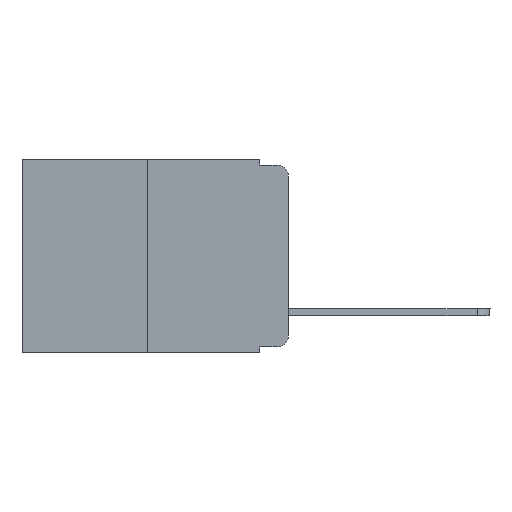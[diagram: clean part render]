
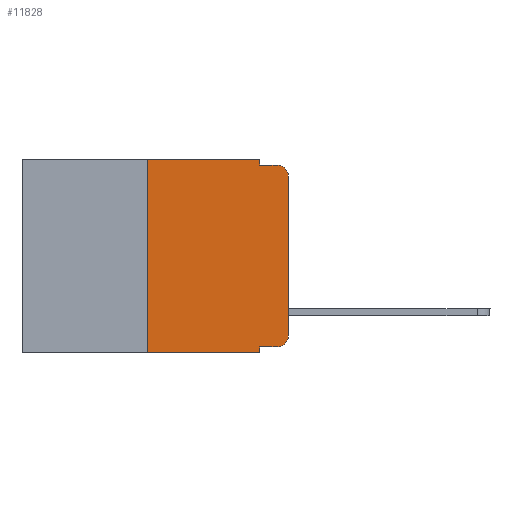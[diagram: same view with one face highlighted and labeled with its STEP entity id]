
A CAD part, left-side view. The second image highlights one B-rep face of the part: STEP entity #11828.
In plain terms, the highlighted planar face has unit normal (-1, 0, 0).
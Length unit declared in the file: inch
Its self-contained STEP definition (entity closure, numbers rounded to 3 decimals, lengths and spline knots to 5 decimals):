
#53 = LINE ( 'NONE', #4041, #8085 ) ;
#580 = ORIENTED_EDGE ( 'NONE', *, *, #9671, .T. ) ;
#917 = ORIENTED_EDGE ( 'NONE', *, *, #2712, .T. ) ;
#971 = VERTEX_POINT ( 'NONE', #9948 ) ;
#1111 = DIRECTION ( 'NONE',  ( 0., 0., -1. ) ) ;
#1270 = VERTEX_POINT ( 'NONE', #3355 ) ;
#1371 = PLANE ( 'NONE',  #2967 ) ;
#1512 = DIRECTION ( 'NONE',  ( -1., 0., 0. ) ) ;
#1575 = CARTESIAN_POINT ( 'NONE',  ( 0., 0.25, 0. ) ) ;
#1834 = VERTEX_POINT ( 'NONE', #2015 ) ;
#1942 = ORIENTED_EDGE ( 'NONE', *, *, #8158, .F. ) ;
#2015 = CARTESIAN_POINT ( 'NONE',  ( 0., 0., -0.03 ) ) ;
#2259 = EDGE_CURVE ( 'NONE', #1270, #7392, #3887, .T. ) ;
#2480 = DIRECTION ( 'NONE',  ( 0., -1., 0. ) ) ;
#2538 = ORIENTED_EDGE ( 'NONE', *, *, #11429, .F. ) ;
#2557 = AXIS2_PLACEMENT_3D ( 'NONE', #5615, #1512, #8668 ) ;
#2712 = EDGE_CURVE ( 'NONE', #11240, #7213, #8739, .T. ) ;
#2851 = CARTESIAN_POINT ( 'NONE',  ( 0., 0.02, -0.01 ) ) ;
#2967 = AXIS2_PLACEMENT_3D ( 'NONE', #11277, #10337, #5254 ) ;
#2995 = DIRECTION ( 'NONE',  ( 0., -1., 0. ) ) ;
#3071 = CARTESIAN_POINT ( 'NONE',  ( 0., 0.02, -0.333 ) ) ;
#3355 = CARTESIAN_POINT ( 'NONE',  ( 0., 0.25, 0. ) ) ;
#3543 = CARTESIAN_POINT ( 'NONE',  ( 0., 0.051, 0. ) ) ;
#3721 = ORIENTED_EDGE ( 'NONE', *, *, #9309, .T. ) ;
#3887 = LINE ( 'NONE', #11748, #8370 ) ;
#4041 = CARTESIAN_POINT ( 'NONE',  ( 0., 0.051, 0. ) ) ;
#4401 = LINE ( 'NONE', #1575, #8736 ) ;
#4431 = VECTOR ( 'NONE', #11835, 39.37008 ) ;
#4717 = CARTESIAN_POINT ( 'NONE',  ( 0., 0.051, -0.333 ) ) ;
#4835 = CIRCLE ( 'NONE', #7075, 0.02 ) ;
#4904 = CARTESIAN_POINT ( 'NONE',  ( 0., 0.051, -0.343 ) ) ;
#5161 = CARTESIAN_POINT ( 'NONE',  ( 0., 0.02, -0.313 ) ) ;
#5254 = DIRECTION ( 'NONE',  ( 0., 0., -1. ) ) ;
#5384 = LINE ( 'NONE', #3543, #12582 ) ;
#5615 = CARTESIAN_POINT ( 'NONE',  ( 0., 0.02, -0.03 ) ) ;
#5654 = VECTOR ( 'NONE', #7836, 39.37008 ) ;
#5767 = VERTEX_POINT ( 'NONE', #4904 ) ;
#5977 = CARTESIAN_POINT ( 'NONE',  ( 0., 0.473, -0.343 ) ) ;
#6261 = EDGE_CURVE ( 'NONE', #11240, #5767, #53, .T. ) ;
#6270 = VECTOR ( 'NONE', #2480, 39.37008 ) ;
#6350 = FACE_OUTER_BOUND ( 'NONE', #10486, .T. ) ;
#6461 = VECTOR ( 'NONE', #2995, 39.37008 ) ;
#7012 = VERTEX_POINT ( 'NONE', #9986 ) ;
#7075 = AXIS2_PLACEMENT_3D ( 'NONE', #5161, #7221, #1111 ) ;
#7213 = VERTEX_POINT ( 'NONE', #3071 ) ;
#7221 = DIRECTION ( 'NONE',  ( -1., 0., 0. ) ) ;
#7392 = VERTEX_POINT ( 'NONE', #7744 ) ;
#7400 = LINE ( 'NONE', #8438, #6270 ) ;
#7733 = EDGE_CURVE ( 'NONE', #12486, #11244, #7400, .T. ) ;
#7744 = CARTESIAN_POINT ( 'NONE',  ( 0., 0.051, 0. ) ) ;
#7836 = DIRECTION ( 'NONE',  ( 0., -1., 0. ) ) ;
#7876 = ORIENTED_EDGE ( 'NONE', *, *, #6261, .F. ) ;
#7999 = DIRECTION ( 'NONE',  ( 0., 0., -1. ) ) ;
#8085 = VECTOR ( 'NONE', #7999, 39.37008 ) ;
#8158 = EDGE_CURVE ( 'NONE', #7012, #1270, #4401, .T. ) ;
#8370 = VECTOR ( 'NONE', #11873, 39.37008 ) ;
#8438 = CARTESIAN_POINT ( 'NONE',  ( 0., 0.051, -0.01 ) ) ;
#8668 = DIRECTION ( 'NONE',  ( 0., 0., -1. ) ) ;
#8736 = VECTOR ( 'NONE', #9485, 39.37008 ) ;
#8739 = LINE ( 'NONE', #4717, #5654 ) ;
#9098 = EDGE_CURVE ( 'NONE', #1834, #11244, #9596, .T. ) ;
#9309 = EDGE_CURVE ( 'NONE', #7213, #971, #4835, .T. ) ;
#9485 = DIRECTION ( 'NONE',  ( 0., 0., 1. ) ) ;
#9596 = CIRCLE ( 'NONE', #2557, 0.02 ) ;
#9671 = EDGE_CURVE ( 'NONE', #7012, #5767, #12027, .T. ) ;
#9854 = LINE ( 'NONE', #12035, #4431 ) ;
#9948 = CARTESIAN_POINT ( 'NONE',  ( 0., 0., -0.313 ) ) ;
#9986 = CARTESIAN_POINT ( 'NONE',  ( 0., 0.25, -0.343 ) ) ;
#10302 = ORIENTED_EDGE ( 'NONE', *, *, #7733, .F. ) ;
#10337 = DIRECTION ( 'NONE',  ( 1., 0., 0. ) ) ;
#10486 = EDGE_LOOP ( 'NONE', ( #12150, #11140, #10302, #2538, #12808, #1942, #580, #7876, #917, #3721 ) ) ;
#10977 = CARTESIAN_POINT ( 'NONE',  ( 0., 0.051, -0.01 ) ) ;
#11140 = ORIENTED_EDGE ( 'NONE', *, *, #9098, .T. ) ;
#11240 = VERTEX_POINT ( 'NONE', #11817 ) ;
#11244 = VERTEX_POINT ( 'NONE', #2851 ) ;
#11277 = CARTESIAN_POINT ( 'NONE',  ( 0., 0.473, 0. ) ) ;
#11407 = DIRECTION ( 'NONE',  ( 0., 0., -1. ) ) ;
#11429 = EDGE_CURVE ( 'NONE', #7392, #12486, #5384, .T. ) ;
#11748 = CARTESIAN_POINT ( 'NONE',  ( 0., 0.473, 0. ) ) ;
#11817 = CARTESIAN_POINT ( 'NONE',  ( 0., 0.051, -0.333 ) ) ;
#11828 = ADVANCED_FACE ( 'NONE', ( #6350 ), #1371, .F. ) ;
#11835 = DIRECTION ( 'NONE',  ( 0., 0., 1. ) ) ;
#11873 = DIRECTION ( 'NONE',  ( 0., -1., 0. ) ) ;
#12027 = LINE ( 'NONE', #5977, #6461 ) ;
#12035 = CARTESIAN_POINT ( 'NONE',  ( 0., 0., 0. ) ) ;
#12150 = ORIENTED_EDGE ( 'NONE', *, *, #12547, .T. ) ;
#12486 = VERTEX_POINT ( 'NONE', #10977 ) ;
#12547 = EDGE_CURVE ( 'NONE', #971, #1834, #9854, .T. ) ;
#12582 = VECTOR ( 'NONE', #11407, 39.37008 ) ;
#12808 = ORIENTED_EDGE ( 'NONE', *, *, #2259, .F. ) ;
